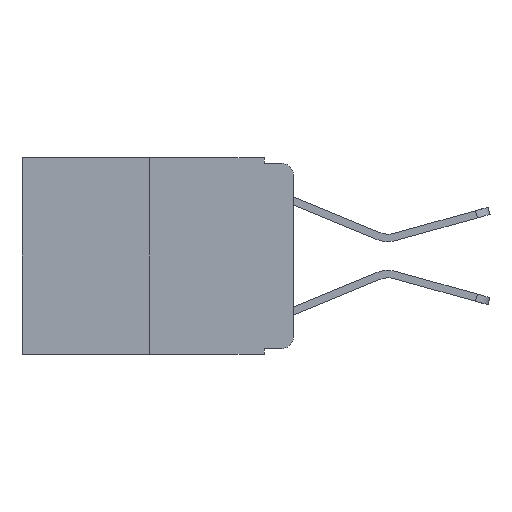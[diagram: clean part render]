
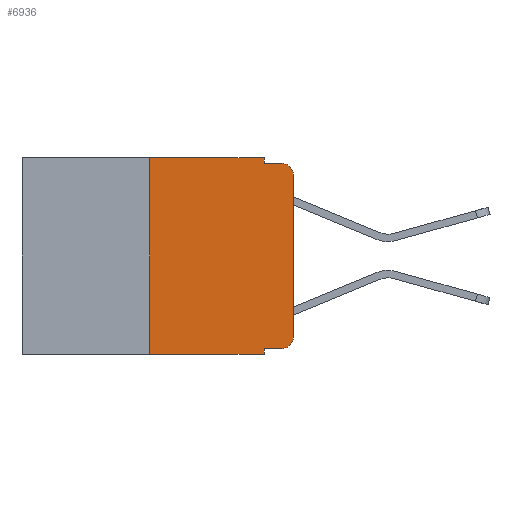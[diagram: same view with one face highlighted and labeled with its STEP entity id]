
A CAD part, left-side view. The second image highlights one B-rep face of the part: STEP entity #6936.
In plain terms, the highlighted planar face has unit normal (-1, 0, 0).
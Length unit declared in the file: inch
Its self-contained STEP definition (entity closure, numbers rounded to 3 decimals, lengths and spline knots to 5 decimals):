
#271 = VERTEX_POINT ( 'NONE', #10669 ) ;
#399 = EDGE_LOOP ( 'NONE', ( #566, #5927, #3700, #8725, #6753, #11339, #7572, #7826, #752, #6076 ) ) ;
#501 = VECTOR ( 'NONE', #8061, 39.37008 ) ;
#566 = ORIENTED_EDGE ( 'NONE', *, *, #6324, .T. ) ;
#752 = ORIENTED_EDGE ( 'NONE', *, *, #2486, .T. ) ;
#784 = VECTOR ( 'NONE', #5376, 39.37008 ) ;
#1001 = LINE ( 'NONE', #8168, #6552 ) ;
#1223 = VERTEX_POINT ( 'NONE', #2670 ) ;
#1387 = LINE ( 'NONE', #4336, #10676 ) ;
#1729 = LINE ( 'NONE', #11702, #4103 ) ;
#1757 = EDGE_CURVE ( 'NONE', #7695, #6865, #10448, .T. ) ;
#1761 = CARTESIAN_POINT ( 'NONE',  ( 0., 0., -0.313 ) ) ;
#2206 = DIRECTION ( 'NONE',  ( 0., 0., -1. ) ) ;
#2207 = DIRECTION ( 'NONE',  ( -1., 0., 0. ) ) ;
#2230 = DIRECTION ( 'NONE',  ( -1., 0., 0. ) ) ;
#2407 = EDGE_CURVE ( 'NONE', #7181, #10197, #10307, .T. ) ;
#2486 = EDGE_CURVE ( 'NONE', #4698, #7695, #1387, .T. ) ;
#2670 = CARTESIAN_POINT ( 'NONE',  ( 0., 0.25, -0.343 ) ) ;
#2839 = DIRECTION ( 'NONE',  ( 0., 0., 1. ) ) ;
#2955 = CIRCLE ( 'NONE', #6965, 0.02 ) ;
#3154 = EDGE_CURVE ( 'NONE', #4698, #271, #1001, .T. ) ;
#3178 = CARTESIAN_POINT ( 'NONE',  ( 0., 0., 0. ) ) ;
#3211 = CARTESIAN_POINT ( 'NONE',  ( 0., 0.051, -0.01 ) ) ;
#3464 = CARTESIAN_POINT ( 'NONE',  ( 0., 0.25, 0. ) ) ;
#3582 = LINE ( 'NONE', #5418, #784 ) ;
#3700 = ORIENTED_EDGE ( 'NONE', *, *, #5099, .F. ) ;
#3806 = EDGE_CURVE ( 'NONE', #1223, #7181, #10762, .T. ) ;
#3908 = VECTOR ( 'NONE', #2839, 39.37008 ) ;
#3934 = CARTESIAN_POINT ( 'NONE',  ( 0., 0.473, 0. ) ) ;
#4103 = VECTOR ( 'NONE', #6823, 39.37008 ) ;
#4336 = CARTESIAN_POINT ( 'NONE',  ( 0., 0.051, -0.333 ) ) ;
#4442 = EDGE_CURVE ( 'NONE', #10197, #10849, #3582, .T. ) ;
#4698 = VERTEX_POINT ( 'NONE', #6081 ) ;
#4835 = CARTESIAN_POINT ( 'NONE',  ( 0., 0.051, 0. ) ) ;
#5035 = LINE ( 'NONE', #3178, #7675 ) ;
#5099 = EDGE_CURVE ( 'NONE', #10849, #8189, #10754, .T. ) ;
#5376 = DIRECTION ( 'NONE',  ( 0., 0., -1. ) ) ;
#5418 = CARTESIAN_POINT ( 'NONE',  ( 0., 0.051, 0. ) ) ;
#5480 = AXIS2_PLACEMENT_3D ( 'NONE', #5759, #11543, #6648 ) ;
#5717 = EDGE_CURVE ( 'NONE', #8796, #8189, #2955, .T. ) ;
#5759 = CARTESIAN_POINT ( 'NONE',  ( 0., 0.473, 0. ) ) ;
#5927 = ORIENTED_EDGE ( 'NONE', *, *, #5717, .T. ) ;
#6076 = ORIENTED_EDGE ( 'NONE', *, *, #1757, .T. ) ;
#6081 = CARTESIAN_POINT ( 'NONE',  ( 0., 0.051, -0.333 ) ) ;
#6324 = EDGE_CURVE ( 'NONE', #6865, #8796, #5035, .T. ) ;
#6552 = VECTOR ( 'NONE', #8181, 39.37008 ) ;
#6590 = DIRECTION ( 'NONE',  ( 0., -1., 0. ) ) ;
#6648 = DIRECTION ( 'NONE',  ( 0., 0., -1. ) ) ;
#6753 = ORIENTED_EDGE ( 'NONE', *, *, #2407, .F. ) ;
#6754 = CARTESIAN_POINT ( 'NONE',  ( 0., 0., -0.03 ) ) ;
#6823 = DIRECTION ( 'NONE',  ( 0., -1., 0. ) ) ;
#6865 = VERTEX_POINT ( 'NONE', #1761 ) ;
#6936 = ADVANCED_FACE ( 'NONE', ( #9816 ), #9937, .F. ) ;
#6965 = AXIS2_PLACEMENT_3D ( 'NONE', #7794, #2230, #8618 ) ;
#7181 = VERTEX_POINT ( 'NONE', #10939 ) ;
#7572 = ORIENTED_EDGE ( 'NONE', *, *, #7830, .T. ) ;
#7675 = VECTOR ( 'NONE', #8571, 39.37008 ) ;
#7695 = VERTEX_POINT ( 'NONE', #9997 ) ;
#7794 = CARTESIAN_POINT ( 'NONE',  ( 0., 0.02, -0.03 ) ) ;
#7826 = ORIENTED_EDGE ( 'NONE', *, *, #3154, .F. ) ;
#7830 = EDGE_CURVE ( 'NONE', #1223, #271, #1729, .T. ) ;
#8061 = DIRECTION ( 'NONE',  ( 0., -1., 0. ) ) ;
#8168 = CARTESIAN_POINT ( 'NONE',  ( 0., 0.051, 0. ) ) ;
#8181 = DIRECTION ( 'NONE',  ( 0., 0., -1. ) ) ;
#8189 = VERTEX_POINT ( 'NONE', #11202 ) ;
#8571 = DIRECTION ( 'NONE',  ( 0., 0., 1. ) ) ;
#8618 = DIRECTION ( 'NONE',  ( 0., 0., -1. ) ) ;
#8627 = VECTOR ( 'NONE', #9451, 39.37008 ) ;
#8725 = ORIENTED_EDGE ( 'NONE', *, *, #4442, .F. ) ;
#8796 = VERTEX_POINT ( 'NONE', #6754 ) ;
#8898 = CARTESIAN_POINT ( 'NONE',  ( 0., 0.02, -0.313 ) ) ;
#9451 = DIRECTION ( 'NONE',  ( 0., -1., 0. ) ) ;
#9763 = CARTESIAN_POINT ( 'NONE',  ( 0., 0.051, -0.01 ) ) ;
#9816 = FACE_OUTER_BOUND ( 'NONE', #399, .T. ) ;
#9937 = PLANE ( 'NONE',  #5480 ) ;
#9997 = CARTESIAN_POINT ( 'NONE',  ( 0., 0.02, -0.333 ) ) ;
#10197 = VERTEX_POINT ( 'NONE', #4835 ) ;
#10307 = LINE ( 'NONE', #3934, #501 ) ;
#10448 = CIRCLE ( 'NONE', #11833, 0.02 ) ;
#10669 = CARTESIAN_POINT ( 'NONE',  ( 0., 0.051, -0.343 ) ) ;
#10676 = VECTOR ( 'NONE', #6590, 39.37008 ) ;
#10754 = LINE ( 'NONE', #3211, #8627 ) ;
#10762 = LINE ( 'NONE', #3464, #3908 ) ;
#10849 = VERTEX_POINT ( 'NONE', #9763 ) ;
#10939 = CARTESIAN_POINT ( 'NONE',  ( 0., 0.25, 0. ) ) ;
#11202 = CARTESIAN_POINT ( 'NONE',  ( 0., 0.02, -0.01 ) ) ;
#11339 = ORIENTED_EDGE ( 'NONE', *, *, #3806, .F. ) ;
#11543 = DIRECTION ( 'NONE',  ( 1., 0., 0. ) ) ;
#11702 = CARTESIAN_POINT ( 'NONE',  ( 0., 0.473, -0.343 ) ) ;
#11833 = AXIS2_PLACEMENT_3D ( 'NONE', #8898, #2207, #2206 ) ;
